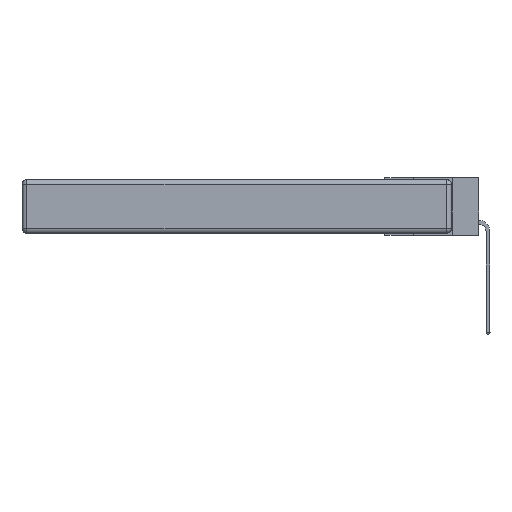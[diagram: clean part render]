
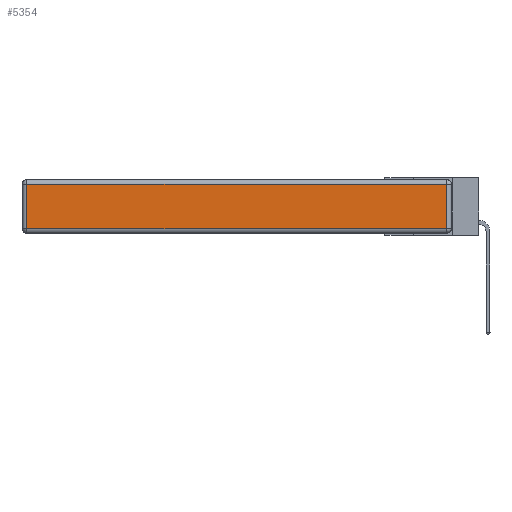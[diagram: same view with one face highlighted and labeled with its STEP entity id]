
A CAD part, left-side view. The second image highlights one B-rep face of the part: STEP entity #5354.
In plain terms, the highlighted planar face has unit normal (-1, 0, 0).
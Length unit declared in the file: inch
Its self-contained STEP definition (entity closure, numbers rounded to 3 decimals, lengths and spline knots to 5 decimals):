
#724 = VECTOR ( 'NONE', #17939, 39.37008 ) ;
#945 = DIRECTION ( 'NONE',  ( 0., 0., -1. ) ) ;
#2208 = VECTOR ( 'NONE', #15352, 39.37008 ) ;
#3710 = VERTEX_POINT ( 'NONE', #14502 ) ;
#3893 = DIRECTION ( 'NONE',  ( 0., 0., 1. ) ) ;
#4170 = LINE ( 'NONE', #4922, #17771 ) ;
#4530 = CARTESIAN_POINT ( 'NONE',  ( 0., 0.03, -0.03 ) ) ;
#4767 = VERTEX_POINT ( 'NONE', #21231 ) ;
#4922 = CARTESIAN_POINT ( 'NONE',  ( 0., 2.72, -0.343 ) ) ;
#5203 = ORIENTED_EDGE ( 'NONE', *, *, #17614, .T. ) ;
#5354 = ADVANCED_FACE ( 'NONE', ( #11969 ), #16028, .T. ) ;
#6881 = VERTEX_POINT ( 'NONE', #4530 ) ;
#7715 = LINE ( 'NONE', #21667, #724 ) ;
#7912 = EDGE_LOOP ( 'NONE', ( #8192, #18482, #5203, #10599 ) ) ;
#8192 = ORIENTED_EDGE ( 'NONE', *, *, #19755, .T. ) ;
#8836 = LINE ( 'NONE', #25444, #10123 ) ;
#8990 = CARTESIAN_POINT ( 'NONE',  ( 0., 0.03, -0.343 ) ) ;
#10123 = VECTOR ( 'NONE', #19196, 39.37008 ) ;
#10595 = EDGE_CURVE ( 'NONE', #4767, #6881, #24383, .T. ) ;
#10599 = ORIENTED_EDGE ( 'NONE', *, *, #23353, .T. ) ;
#11969 = FACE_OUTER_BOUND ( 'NONE', #7912, .T. ) ;
#14341 = CARTESIAN_POINT ( 'NONE',  ( 0., 2.72, -0.03 ) ) ;
#14502 = CARTESIAN_POINT ( 'NONE',  ( 0., 2.72, -0.313 ) ) ;
#15352 = DIRECTION ( 'NONE',  ( 0., 0., 1. ) ) ;
#15765 = DIRECTION ( 'NONE',  ( -1., 0., 0. ) ) ;
#15855 = CARTESIAN_POINT ( 'NONE',  ( 0., 0., -0.343 ) ) ;
#16028 = PLANE ( 'NONE',  #25149 ) ;
#17614 = EDGE_CURVE ( 'NONE', #6881, #25574, #7715, .T. ) ;
#17771 = VECTOR ( 'NONE', #945, 39.37008 ) ;
#17939 = DIRECTION ( 'NONE',  ( 0., 1., 0. ) ) ;
#18482 = ORIENTED_EDGE ( 'NONE', *, *, #10595, .T. ) ;
#19196 = DIRECTION ( 'NONE',  ( 0., -1., 0. ) ) ;
#19755 = EDGE_CURVE ( 'NONE', #3710, #4767, #8836, .T. ) ;
#21231 = CARTESIAN_POINT ( 'NONE',  ( 0., 0.03, -0.313 ) ) ;
#21667 = CARTESIAN_POINT ( 'NONE',  ( 0., 2.75, -0.03 ) ) ;
#23353 = EDGE_CURVE ( 'NONE', #25574, #3710, #4170, .T. ) ;
#24383 = LINE ( 'NONE', #8990, #2208 ) ;
#25149 = AXIS2_PLACEMENT_3D ( 'NONE', #15855, #15765, #3893 ) ;
#25444 = CARTESIAN_POINT ( 'NONE',  ( 0., 0., -0.313 ) ) ;
#25574 = VERTEX_POINT ( 'NONE', #14341 ) ;
